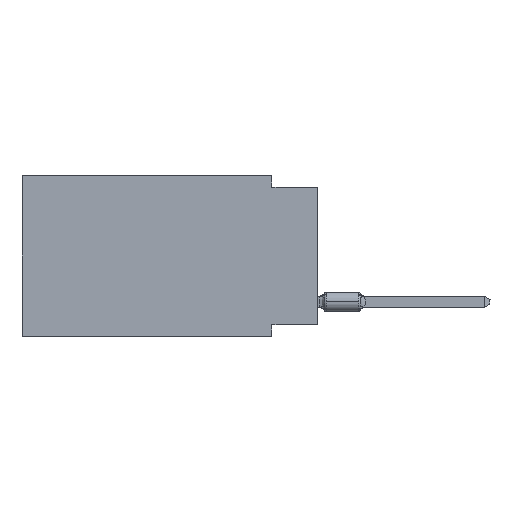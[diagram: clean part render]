
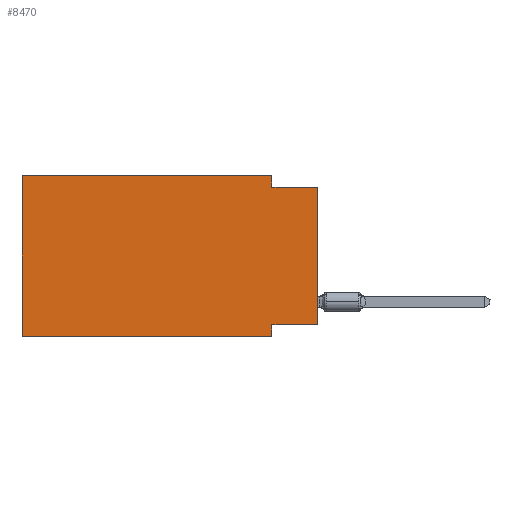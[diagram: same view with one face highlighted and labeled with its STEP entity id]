
A CAD part, left-side view. The second image highlights one B-rep face of the part: STEP entity #8470.
In plain terms, the highlighted planar face has unit normal (-1, 0, 0).
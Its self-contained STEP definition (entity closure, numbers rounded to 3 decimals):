
#1272 = CARTESIAN_POINT ( 'NONE',  ( 0., 16.383, 0. ) ) ;
#1840 = ORIENTED_EDGE ( 'NONE', *, *, #38033, .F. ) ;
#2250 = EDGE_CURVE ( 'NONE', #67536, #72126, #76634, .T. ) ;
#2842 = VERTEX_POINT ( 'NONE', #13561 ) ;
#3815 = EDGE_CURVE ( 'NONE', #6913, #67536, #9097, .T. ) ;
#5365 = DIRECTION ( 'NONE',  ( 0., -1., 0. ) ) ;
#6913 = VERTEX_POINT ( 'NONE', #1272 ) ;
#7193 = CARTESIAN_POINT ( 'NONE',  ( 0., 2.54, -0.635 ) ) ;
#7908 = LINE ( 'NONE', #14327, #22952 ) ;
#8470 = ADVANCED_FACE ( 'NONE', ( #17965 ), #77327, .F. ) ;
#8947 = VERTEX_POINT ( 'NONE', #75151 ) ;
#9097 = LINE ( 'NONE', #9522, #31837 ) ;
#9522 = CARTESIAN_POINT ( 'NONE',  ( 0., 16.383, 0. ) ) ;
#10434 = DIRECTION ( 'NONE',  ( 0., 0., -1. ) ) ;
#10436 = VECTOR ( 'NONE', #5365, 1000. ) ;
#12524 = EDGE_CURVE ( 'NONE', #81696, #2842, #13292, .T. ) ;
#13292 = LINE ( 'NONE', #32519, #65419 ) ;
#13561 = CARTESIAN_POINT ( 'NONE',  ( 0., 0., -0.635 ) ) ;
#14327 = CARTESIAN_POINT ( 'NONE',  ( 0., 0., -8.255 ) ) ;
#16977 = ORIENTED_EDGE ( 'NONE', *, *, #3815, .F. ) ;
#17113 = CARTESIAN_POINT ( 'NONE',  ( 0., 16.383, 0. ) ) ;
#17965 = FACE_OUTER_BOUND ( 'NONE', #36541, .T. ) ;
#19486 = CARTESIAN_POINT ( 'NONE',  ( 0., 16.383, -8.89 ) ) ;
#21178 = CARTESIAN_POINT ( 'NONE',  ( 0., 0., -0.635 ) ) ;
#22952 = VECTOR ( 'NONE', #66875, 1000. ) ;
#23961 = VERTEX_POINT ( 'NONE', #31239 ) ;
#25022 = LINE ( 'NONE', #31407, #10436 ) ;
#25255 = CARTESIAN_POINT ( 'NONE',  ( 0., 2.54, -8.89 ) ) ;
#29529 = ORIENTED_EDGE ( 'NONE', *, *, #47123, .F. ) ;
#30896 = EDGE_CURVE ( 'NONE', #23961, #8947, #70969, .T. ) ;
#31239 = CARTESIAN_POINT ( 'NONE',  ( 0., 2.54, -8.255 ) ) ;
#31407 = CARTESIAN_POINT ( 'NONE',  ( 0., 16.383, -8.89 ) ) ;
#31837 = VECTOR ( 'NONE', #35133, 1000. ) ;
#32156 = ORIENTED_EDGE ( 'NONE', *, *, #12524, .T. ) ;
#32519 = CARTESIAN_POINT ( 'NONE',  ( 0., 0., 0. ) ) ;
#32728 = CARTESIAN_POINT ( 'NONE',  ( 0., 0., -8.255 ) ) ;
#34103 = CARTESIAN_POINT ( 'NONE',  ( 0., 16.383, 0. ) ) ;
#35133 = DIRECTION ( 'NONE',  ( 0., -1., 0. ) ) ;
#35725 = EDGE_CURVE ( 'NONE', #72126, #2842, #67718, .T. ) ;
#36541 = EDGE_LOOP ( 'NONE', ( #32156, #80783, #51897, #16977, #1840, #77466, #75264, #29529 ) ) ;
#37597 = DIRECTION ( 'NONE',  ( 1., 0., 0. ) ) ;
#38033 = EDGE_CURVE ( 'NONE', #44758, #6913, #54171, .T. ) ;
#41358 = CARTESIAN_POINT ( 'NONE',  ( 0., 2.54, 0. ) ) ;
#43280 = DIRECTION ( 'NONE',  ( 0., 0., -1. ) ) ;
#44147 = CARTESIAN_POINT ( 'NONE',  ( 0., 2.54, 0. ) ) ;
#44758 = VERTEX_POINT ( 'NONE', #19486 ) ;
#46512 = DIRECTION ( 'NONE',  ( 0., 0., 1. ) ) ;
#46584 = VECTOR ( 'NONE', #48079, 1000. ) ;
#47123 = EDGE_CURVE ( 'NONE', #81696, #23961, #7908, .T. ) ;
#48079 = DIRECTION ( 'NONE',  ( 0., -1., 0. ) ) ;
#51763 = DIRECTION ( 'NONE',  ( 0., 0., 1. ) ) ;
#51897 = ORIENTED_EDGE ( 'NONE', *, *, #2250, .F. ) ;
#54171 = LINE ( 'NONE', #34103, #66047 ) ;
#56157 = EDGE_CURVE ( 'NONE', #44758, #8947, #25022, .T. ) ;
#56273 = VECTOR ( 'NONE', #10434, 1000. ) ;
#57690 = DIRECTION ( 'NONE',  ( 0., 0., -1. ) ) ;
#65419 = VECTOR ( 'NONE', #51763, 1000. ) ;
#66047 = VECTOR ( 'NONE', #46512, 1000. ) ;
#66875 = DIRECTION ( 'NONE',  ( 0., 1., 0. ) ) ;
#67536 = VERTEX_POINT ( 'NONE', #41358 ) ;
#67718 = LINE ( 'NONE', #21178, #46584 ) ;
#70969 = LINE ( 'NONE', #25255, #56273 ) ;
#72126 = VERTEX_POINT ( 'NONE', #7193 ) ;
#73307 = AXIS2_PLACEMENT_3D ( 'NONE', #17113, #37597, #57690 ) ;
#75151 = CARTESIAN_POINT ( 'NONE',  ( 0., 2.54, -8.89 ) ) ;
#75264 = ORIENTED_EDGE ( 'NONE', *, *, #30896, .F. ) ;
#76634 = LINE ( 'NONE', #44147, #82365 ) ;
#77327 = PLANE ( 'NONE',  #73307 ) ;
#77466 = ORIENTED_EDGE ( 'NONE', *, *, #56157, .T. ) ;
#80783 = ORIENTED_EDGE ( 'NONE', *, *, #35725, .F. ) ;
#81696 = VERTEX_POINT ( 'NONE', #32728 ) ;
#82365 = VECTOR ( 'NONE', #43280, 1000. ) ;
